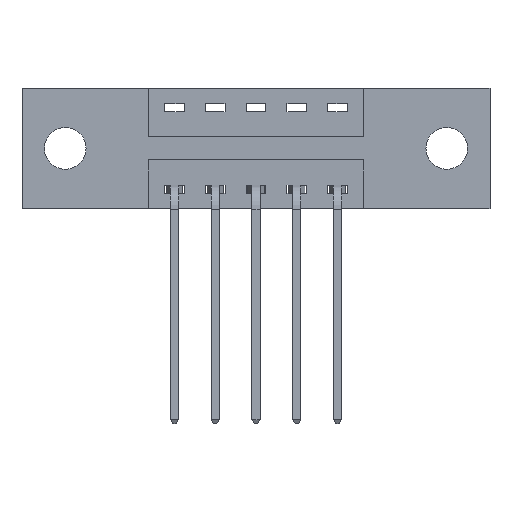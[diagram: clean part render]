
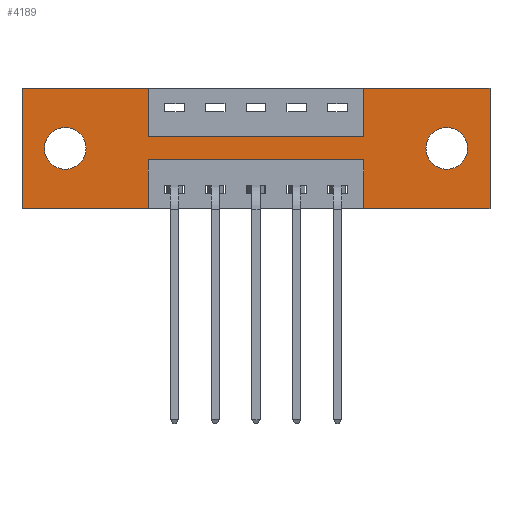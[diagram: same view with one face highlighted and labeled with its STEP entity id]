
A CAD part, front view. The second image highlights one B-rep face of the part: STEP entity #4189.
In plain terms, the highlighted planar face has unit normal (0, -1, 0).
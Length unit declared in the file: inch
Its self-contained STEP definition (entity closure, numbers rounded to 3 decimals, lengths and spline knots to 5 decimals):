
#6 = VERTEX_POINT ( 'NONE', #387 ) ;
#187 = CARTESIAN_POINT ( 'NONE',  ( 0.3875, 0., 0. ) ) ;
#350 = CARTESIAN_POINT ( 'NONE',  ( 1.0475, 0., 0. ) ) ;
#371 = CARTESIAN_POINT ( 'NONE',  ( 0., 0., 0. ) ) ;
#373 = CIRCLE ( 'NONE', #7051, 0.064 ) ;
#387 = CARTESIAN_POINT ( 'NONE',  ( 0.3875, 0., -0.15 ) ) ;
#476 = VERTEX_POINT ( 'NONE', #2490 ) ;
#529 = DIRECTION ( 'NONE',  ( 1., 0., 0. ) ) ;
#610 = EDGE_LOOP ( 'NONE', ( #6032, #5671, #5655, #5544, #6520, #6981, #7372, #6430, #5528, #5479, #6599, #4158 ) ) ;
#795 = CARTESIAN_POINT ( 'NONE',  ( 1.3025, 0., -0.185 ) ) ;
#840 = VERTEX_POINT ( 'NONE', #2843 ) ;
#909 = VERTEX_POINT ( 'NONE', #5535 ) ;
#1062 = VERTEX_POINT ( 'NONE', #5925 ) ;
#1116 = VECTOR ( 'NONE', #1158, 39.37008 ) ;
#1158 = DIRECTION ( 'NONE',  ( 1., 0., 0. ) ) ;
#1227 = EDGE_LOOP ( 'NONE', ( #4376, #4367 ) ) ;
#1277 = VECTOR ( 'NONE', #1327, 39.37008 ) ;
#1278 = AXIS2_PLACEMENT_3D ( 'NONE', #3371, #3343, #8188 ) ;
#1302 = VERTEX_POINT ( 'NONE', #6352 ) ;
#1327 = DIRECTION ( 'NONE',  ( -1., 0., 0. ) ) ;
#1358 = CARTESIAN_POINT ( 'NONE',  ( 0., 0., -0.37 ) ) ;
#1361 = LINE ( 'NONE', #371, #1116 ) ;
#1383 = VECTOR ( 'NONE', #2448, 39.37008 ) ;
#1512 = CIRCLE ( 'NONE', #7288, 0.064 ) ;
#1551 = DIRECTION ( 'NONE',  ( 0., 0., -1. ) ) ;
#1649 = VECTOR ( 'NONE', #7166, 39.37008 ) ;
#1742 = VERTEX_POINT ( 'NONE', #7154 ) ;
#1758 = CARTESIAN_POINT ( 'NONE',  ( 0., 0., 0. ) ) ;
#1861 = VERTEX_POINT ( 'NONE', #7675 ) ;
#1940 = VECTOR ( 'NONE', #3440, 39.37008 ) ;
#2026 = DIRECTION ( 'NONE',  ( 0., 1., 0. ) ) ;
#2052 = FACE_OUTER_BOUND ( 'NONE', #610, .T. ) ;
#2214 = CARTESIAN_POINT ( 'NONE',  ( 0., 0., -0.37 ) ) ;
#2253 = AXIS2_PLACEMENT_3D ( 'NONE', #795, #5348, #1551 ) ;
#2272 = VECTOR ( 'NONE', #3067, 39.37008 ) ;
#2276 = EDGE_CURVE ( 'NONE', #6, #2380, #2812, .T. ) ;
#2316 = LINE ( 'NONE', #4677, #1940 ) ;
#2380 = VERTEX_POINT ( 'NONE', #4732 ) ;
#2448 = DIRECTION ( 'NONE',  ( -1., 0., 0. ) ) ;
#2490 = CARTESIAN_POINT ( 'NONE',  ( 1.0475, 0., -0.22 ) ) ;
#2755 = PLANE ( 'NONE',  #1278 ) ;
#2757 = VECTOR ( 'NONE', #6741, 39.37008 ) ;
#2809 = CARTESIAN_POINT ( 'NONE',  ( 1.435, 0., 0. ) ) ;
#2812 = LINE ( 'NONE', #3026, #7351 ) ;
#2839 = VECTOR ( 'NONE', #7576, 39.37008 ) ;
#2843 = CARTESIAN_POINT ( 'NONE',  ( 1.0475, 0., -0.37 ) ) ;
#2931 = EDGE_CURVE ( 'NONE', #1062, #1302, #3672, .T. ) ;
#2942 = EDGE_CURVE ( 'NONE', #7650, #5536, #5199, .T. ) ;
#3009 = VERTEX_POINT ( 'NONE', #5920 ) ;
#3025 = VERTEX_POINT ( 'NONE', #2214 ) ;
#3026 = CARTESIAN_POINT ( 'NONE',  ( 0.3875, 0., -0.15 ) ) ;
#3041 = LINE ( 'NONE', #5610, #1383 ) ;
#3067 = DIRECTION ( 'NONE',  ( 0., 0., 1. ) ) ;
#3148 = EDGE_CURVE ( 'NONE', #840, #476, #7948, .T. ) ;
#3181 = VERTEX_POINT ( 'NONE', #4473 ) ;
#3343 = DIRECTION ( 'NONE',  ( 0., -1., 0. ) ) ;
#3353 = CIRCLE ( 'NONE', #2253, 0.064 ) ;
#3371 = CARTESIAN_POINT ( 'NONE',  ( 0., 0., -0.37 ) ) ;
#3440 = DIRECTION ( 'NONE',  ( 0., 0., -1. ) ) ;
#3550 = CARTESIAN_POINT ( 'NONE',  ( 1.0475, 0., 0. ) ) ;
#3605 = VERTEX_POINT ( 'NONE', #187 ) ;
#3672 = LINE ( 'NONE', #7642, #7005 ) ;
#3788 = CARTESIAN_POINT ( 'NONE',  ( 0.1325, 0., -0.185 ) ) ;
#3815 = CARTESIAN_POINT ( 'NONE',  ( 0.1325, 0., -0.185 ) ) ;
#3886 = FACE_BOUND ( 'NONE', #7698, .T. ) ;
#4158 = ORIENTED_EDGE ( 'NONE', *, *, #5565, .F. ) ;
#4179 = ORIENTED_EDGE ( 'NONE', *, *, #7974, .T. ) ;
#4189 = ADVANCED_FACE ( 'NONE', ( #5405, #3886, #2052 ), #2755, .T. ) ;
#4207 = EDGE_CURVE ( 'NONE', #5536, #5741, #6494, .T. ) ;
#4339 = ORIENTED_EDGE ( 'NONE', *, *, #8014, .T. ) ;
#4367 = ORIENTED_EDGE ( 'NONE', *, *, #5896, .T. ) ;
#4376 = ORIENTED_EDGE ( 'NONE', *, *, #5564, .T. ) ;
#4421 = DIRECTION ( 'NONE',  ( 0., 0., 1. ) ) ;
#4452 = DIRECTION ( 'NONE',  ( 0., 0., 1. ) ) ;
#4473 = CARTESIAN_POINT ( 'NONE',  ( 0., 0., 0. ) ) ;
#4646 = LINE ( 'NONE', #1358, #1277 ) ;
#4677 = CARTESIAN_POINT ( 'NONE',  ( 0.3875, 0., 0. ) ) ;
#4732 = CARTESIAN_POINT ( 'NONE',  ( 1.0475, 0., -0.15 ) ) ;
#4781 = CARTESIAN_POINT ( 'NONE',  ( 1.0475, 0., -0.37 ) ) ;
#4842 = DIRECTION ( 'NONE',  ( 0., 0., 1. ) ) ;
#4918 = EDGE_CURVE ( 'NONE', #3605, #6, #2316, .T. ) ;
#5199 = LINE ( 'NONE', #7593, #2839 ) ;
#5348 = DIRECTION ( 'NONE',  ( 0., 1., 0. ) ) ;
#5405 = FACE_BOUND ( 'NONE', #1227, .T. ) ;
#5436 = CIRCLE ( 'NONE', #7408, 0.064 ) ;
#5479 = ORIENTED_EDGE ( 'NONE', *, *, #7875, .F. ) ;
#5528 = ORIENTED_EDGE ( 'NONE', *, *, #4918, .F. ) ;
#5535 = CARTESIAN_POINT ( 'NONE',  ( 1.3025, 0., -0.121 ) ) ;
#5536 = VERTEX_POINT ( 'NONE', #7480 ) ;
#5544 = ORIENTED_EDGE ( 'NONE', *, *, #6957, .F. ) ;
#5564 = EDGE_CURVE ( 'NONE', #909, #1861, #1512, .T. ) ;
#5565 = EDGE_CURVE ( 'NONE', #1302, #3025, #4646, .T. ) ;
#5610 = CARTESIAN_POINT ( 'NONE',  ( 0.3875, 0., -0.22 ) ) ;
#5655 = ORIENTED_EDGE ( 'NONE', *, *, #3148, .F. ) ;
#5671 = ORIENTED_EDGE ( 'NONE', *, *, #6072, .F. ) ;
#5734 = LINE ( 'NONE', #1758, #2757 ) ;
#5741 = VERTEX_POINT ( 'NONE', #8004 ) ;
#5802 = CARTESIAN_POINT ( 'NONE',  ( 1.3025, 0., -0.185 ) ) ;
#5896 = EDGE_CURVE ( 'NONE', #1861, #909, #3353, .T. ) ;
#5920 = CARTESIAN_POINT ( 'NONE',  ( 0.1325, 0., -0.121 ) ) ;
#5925 = CARTESIAN_POINT ( 'NONE',  ( 0.3875, 0., -0.22 ) ) ;
#6032 = ORIENTED_EDGE ( 'NONE', *, *, #2931, .F. ) ;
#6042 = VECTOR ( 'NONE', #6800, 39.37008 ) ;
#6072 = EDGE_CURVE ( 'NONE', #476, #1062, #3041, .T. ) ;
#6196 = CARTESIAN_POINT ( 'NONE',  ( 0., 0., -0.37 ) ) ;
#6229 = LINE ( 'NONE', #6196, #6042 ) ;
#6352 = CARTESIAN_POINT ( 'NONE',  ( 0.3875, 0., -0.37 ) ) ;
#6430 = ORIENTED_EDGE ( 'NONE', *, *, #2276, .F. ) ;
#6441 = DIRECTION ( 'NONE',  ( 0., 0., -1. ) ) ;
#6494 = LINE ( 'NONE', #2809, #1649 ) ;
#6512 = VECTOR ( 'NONE', #4842, 39.37008 ) ;
#6520 = ORIENTED_EDGE ( 'NONE', *, *, #4207, .F. ) ;
#6599 = ORIENTED_EDGE ( 'NONE', *, *, #7723, .F. ) ;
#6741 = DIRECTION ( 'NONE',  ( 0., 0., 1. ) ) ;
#6800 = DIRECTION ( 'NONE',  ( -1., 0., 0. ) ) ;
#6957 = EDGE_CURVE ( 'NONE', #5741, #840, #6229, .T. ) ;
#6981 = ORIENTED_EDGE ( 'NONE', *, *, #2942, .F. ) ;
#7005 = VECTOR ( 'NONE', #7633, 39.37008 ) ;
#7038 = EDGE_CURVE ( 'NONE', #2380, #7650, #7397, .T. ) ;
#7051 = AXIS2_PLACEMENT_3D ( 'NONE', #3788, #7998, #4421 ) ;
#7154 = CARTESIAN_POINT ( 'NONE',  ( 0.1325, 0., -0.249 ) ) ;
#7166 = DIRECTION ( 'NONE',  ( 0., 0., -1. ) ) ;
#7288 = AXIS2_PLACEMENT_3D ( 'NONE', #5802, #2026, #6441 ) ;
#7351 = VECTOR ( 'NONE', #529, 39.37008 ) ;
#7372 = ORIENTED_EDGE ( 'NONE', *, *, #7038, .F. ) ;
#7397 = LINE ( 'NONE', #350, #2272 ) ;
#7408 = AXIS2_PLACEMENT_3D ( 'NONE', #3815, #8018, #4452 ) ;
#7480 = CARTESIAN_POINT ( 'NONE',  ( 1.435, 0., 0. ) ) ;
#7576 = DIRECTION ( 'NONE',  ( 1., 0., 0. ) ) ;
#7593 = CARTESIAN_POINT ( 'NONE',  ( 0., 0., 0. ) ) ;
#7633 = DIRECTION ( 'NONE',  ( 0., 0., -1. ) ) ;
#7642 = CARTESIAN_POINT ( 'NONE',  ( 0.3875, 0., -0.37 ) ) ;
#7650 = VERTEX_POINT ( 'NONE', #3550 ) ;
#7675 = CARTESIAN_POINT ( 'NONE',  ( 1.3025, 0., -0.249 ) ) ;
#7698 = EDGE_LOOP ( 'NONE', ( #4339, #4179 ) ) ;
#7723 = EDGE_CURVE ( 'NONE', #3025, #3181, #5734, .T. ) ;
#7875 = EDGE_CURVE ( 'NONE', #3181, #3605, #1361, .T. ) ;
#7948 = LINE ( 'NONE', #4781, #6512 ) ;
#7974 = EDGE_CURVE ( 'NONE', #1742, #3009, #373, .T. ) ;
#7998 = DIRECTION ( 'NONE',  ( 0., 1., 0. ) ) ;
#8004 = CARTESIAN_POINT ( 'NONE',  ( 1.435, 0., -0.37 ) ) ;
#8014 = EDGE_CURVE ( 'NONE', #3009, #1742, #5436, .T. ) ;
#8018 = DIRECTION ( 'NONE',  ( 0., 1., 0. ) ) ;
#8188 = DIRECTION ( 'NONE',  ( 0., 0., -1. ) ) ;
